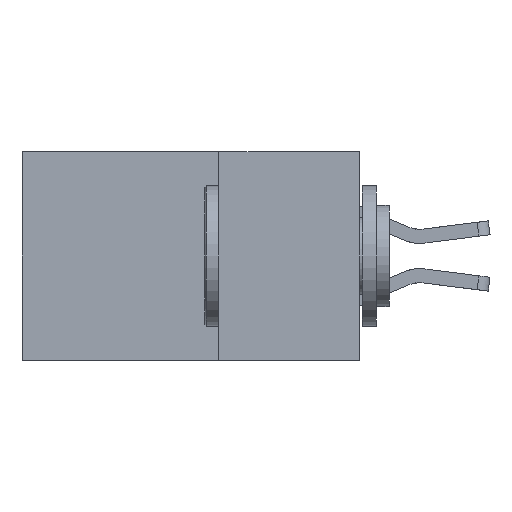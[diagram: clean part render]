
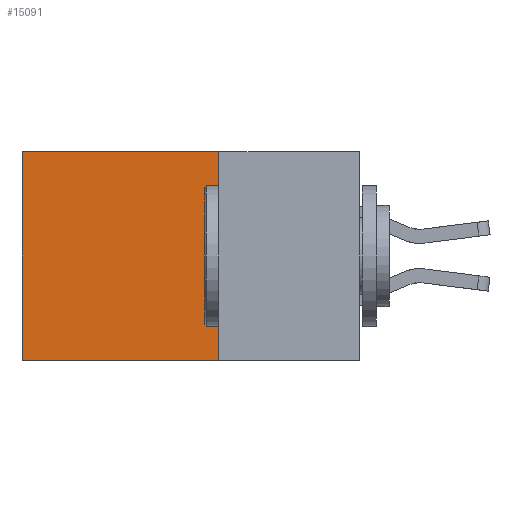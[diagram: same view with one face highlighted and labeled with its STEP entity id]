
A CAD part, left-side view. The second image highlights one B-rep face of the part: STEP entity #15091.
In plain terms, the highlighted planar face has unit normal (-1, 0, 0).
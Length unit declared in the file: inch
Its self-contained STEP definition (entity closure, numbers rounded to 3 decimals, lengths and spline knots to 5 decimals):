
#838 = VERTEX_POINT ( 'NONE', #5842 ) ;
#884 = EDGE_CURVE ( 'NONE', #12455, #13404, #15212, .T. ) ;
#1738 = ORIENTED_EDGE ( 'NONE', *, *, #1881, .T. ) ;
#1750 = VECTOR ( 'NONE', #9149, 39.37008 ) ;
#1881 = EDGE_CURVE ( 'NONE', #14825, #838, #3153, .T. ) ;
#2890 = ORIENTED_EDGE ( 'NONE', *, *, #11406, .F. ) ;
#3153 = LINE ( 'NONE', #8904, #9317 ) ;
#3639 = DIRECTION ( 'NONE',  ( 0., 1., 0. ) ) ;
#4215 = CARTESIAN_POINT ( 'NONE',  ( 0.2875, 0.25, 0. ) ) ;
#4473 = ORIENTED_EDGE ( 'NONE', *, *, #14157, .T. ) ;
#4773 = DIRECTION ( 'NONE',  ( 1., 0., 0. ) ) ;
#4834 = CARTESIAN_POINT ( 'NONE',  ( 0.2875, 0.25, -0.37 ) ) ;
#5239 = CARTESIAN_POINT ( 'NONE',  ( 0.2875, 0.6, 0. ) ) ;
#5842 = CARTESIAN_POINT ( 'NONE',  ( 0.2875, 0.6, 0. ) ) ;
#7765 = FACE_OUTER_BOUND ( 'NONE', #8982, .T. ) ;
#7769 = ORIENTED_EDGE ( 'NONE', *, *, #884, .F. ) ;
#7928 = CARTESIAN_POINT ( 'NONE',  ( 0.2875, 0.25, -0.37 ) ) ;
#8671 = CARTESIAN_POINT ( 'NONE',  ( 0.2875, 0.6, -0.37 ) ) ;
#8678 = DIRECTION ( 'NONE',  ( 0., 1., 0. ) ) ;
#8902 = LINE ( 'NONE', #5239, #14621 ) ;
#8904 = CARTESIAN_POINT ( 'NONE',  ( 0.2875, 0.25, 0. ) ) ;
#8982 = EDGE_LOOP ( 'NONE', ( #4473, #7769, #2890, #1738 ) ) ;
#9149 = DIRECTION ( 'NONE',  ( 0., 0., -1. ) ) ;
#9317 = VECTOR ( 'NONE', #8678, 39.37008 ) ;
#9492 = CARTESIAN_POINT ( 'NONE',  ( 0.2875, 0.25, 0. ) ) ;
#11406 = EDGE_CURVE ( 'NONE', #14825, #12455, #11519, .T. ) ;
#11519 = LINE ( 'NONE', #14833, #1750 ) ;
#11829 = VECTOR ( 'NONE', #3639, 39.37008 ) ;
#11856 = PLANE ( 'NONE',  #15209 ) ;
#12455 = VERTEX_POINT ( 'NONE', #7928 ) ;
#12980 = DIRECTION ( 'NONE',  ( 0., 0., -1. ) ) ;
#13404 = VERTEX_POINT ( 'NONE', #8671 ) ;
#14157 = EDGE_CURVE ( 'NONE', #838, #13404, #8902, .T. ) ;
#14557 = DIRECTION ( 'NONE',  ( 0., 0., -1. ) ) ;
#14621 = VECTOR ( 'NONE', #14557, 39.37008 ) ;
#14825 = VERTEX_POINT ( 'NONE', #4215 ) ;
#14833 = CARTESIAN_POINT ( 'NONE',  ( 0.2875, 0.25, 0. ) ) ;
#15091 = ADVANCED_FACE ( 'NONE', ( #7765 ), #11856, .F. ) ;
#15209 = AXIS2_PLACEMENT_3D ( 'NONE', #9492, #4773, #12980 ) ;
#15212 = LINE ( 'NONE', #4834, #11829 ) ;
